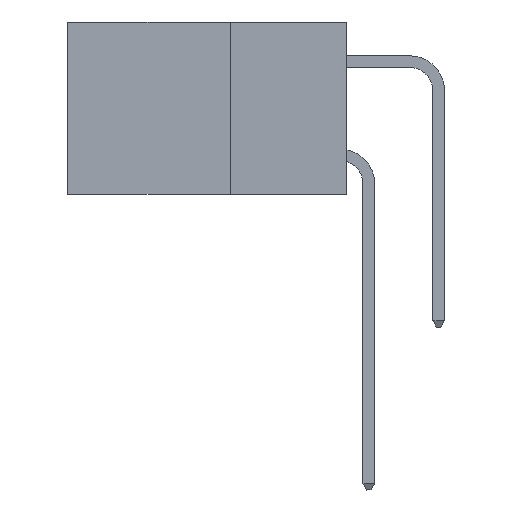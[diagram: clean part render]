
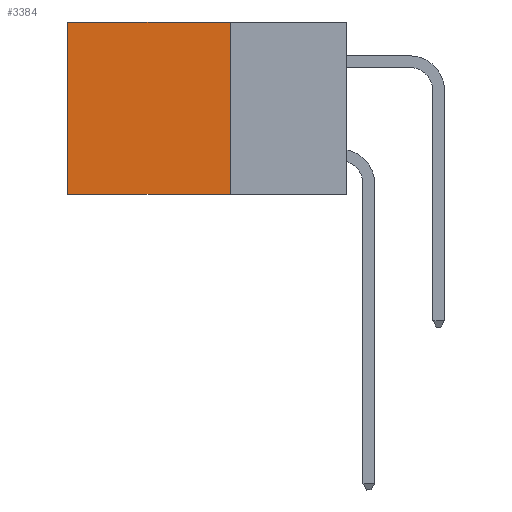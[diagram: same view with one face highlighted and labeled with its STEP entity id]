
A CAD part, left-side view. The second image highlights one B-rep face of the part: STEP entity #3384.
In plain terms, the highlighted planar face has unit normal (-1, 0, 0).
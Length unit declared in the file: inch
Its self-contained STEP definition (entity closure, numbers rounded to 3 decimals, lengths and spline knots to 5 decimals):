
#211 = CARTESIAN_POINT ( 'NONE',  ( 0.2875, 0.6, -0.37 ) ) ;
#615 = CARTESIAN_POINT ( 'NONE',  ( 0.2875, 0.25, 0. ) ) ;
#1646 = CARTESIAN_POINT ( 'NONE',  ( 0.2875, 0.6, 0. ) ) ;
#2244 = DIRECTION ( 'NONE',  ( 0., 0., -1. ) ) ;
#2302 = CARTESIAN_POINT ( 'NONE',  ( 0.2875, 0.25, -0.37 ) ) ;
#3384 = ADVANCED_FACE ( 'NONE', ( #18957 ), #24919, .F. ) ;
#4346 = VECTOR ( 'NONE', #11226, 39.37008 ) ;
#5130 = EDGE_LOOP ( 'NONE', ( #5468, #8277, #15425, #26691 ) ) ;
#5430 = EDGE_CURVE ( 'NONE', #17563, #12882, #13058, .T. ) ;
#5468 = ORIENTED_EDGE ( 'NONE', *, *, #6439, .T. ) ;
#6439 = EDGE_CURVE ( 'NONE', #12882, #10991, #24310, .T. ) ;
#8277 = ORIENTED_EDGE ( 'NONE', *, *, #17530, .F. ) ;
#10708 = VECTOR ( 'NONE', #27369, 39.37008 ) ;
#10910 = DIRECTION ( 'NONE',  ( 0., 1., 0. ) ) ;
#10991 = VERTEX_POINT ( 'NONE', #211 ) ;
#11226 = DIRECTION ( 'NONE',  ( 0., 1., 0. ) ) ;
#12538 = CARTESIAN_POINT ( 'NONE',  ( 0.2875, 0.6, 0. ) ) ;
#12882 = VERTEX_POINT ( 'NONE', #12538 ) ;
#13058 = LINE ( 'NONE', #615, #4346 ) ;
#13873 = CARTESIAN_POINT ( 'NONE',  ( 0.2875, 0.25, 0. ) ) ;
#14964 = VECTOR ( 'NONE', #10910, 39.37008 ) ;
#15318 = VERTEX_POINT ( 'NONE', #25152 ) ;
#15425 = ORIENTED_EDGE ( 'NONE', *, *, #21231, .F. ) ;
#17204 = CARTESIAN_POINT ( 'NONE',  ( 0.2875, 0.25, 0. ) ) ;
#17530 = EDGE_CURVE ( 'NONE', #15318, #10991, #21651, .T. ) ;
#17563 = VERTEX_POINT ( 'NONE', #13873 ) ;
#18667 = CARTESIAN_POINT ( 'NONE',  ( 0.2875, 0.25, 0. ) ) ;
#18957 = FACE_OUTER_BOUND ( 'NONE', #5130, .T. ) ;
#20539 = VECTOR ( 'NONE', #2244, 39.37008 ) ;
#21086 = DIRECTION ( 'NONE',  ( 0., 0., -1. ) ) ;
#21231 = EDGE_CURVE ( 'NONE', #17563, #15318, #24149, .T. ) ;
#21651 = LINE ( 'NONE', #2302, #14964 ) ;
#24149 = LINE ( 'NONE', #17204, #20539 ) ;
#24310 = LINE ( 'NONE', #1646, #10708 ) ;
#24919 = PLANE ( 'NONE',  #25922 ) ;
#25152 = CARTESIAN_POINT ( 'NONE',  ( 0.2875, 0.25, -0.37 ) ) ;
#25922 = AXIS2_PLACEMENT_3D ( 'NONE', #18667, #27320, #21086 ) ;
#26691 = ORIENTED_EDGE ( 'NONE', *, *, #5430, .T. ) ;
#27320 = DIRECTION ( 'NONE',  ( 1., 0., 0. ) ) ;
#27369 = DIRECTION ( 'NONE',  ( 0., 0., -1. ) ) ;
